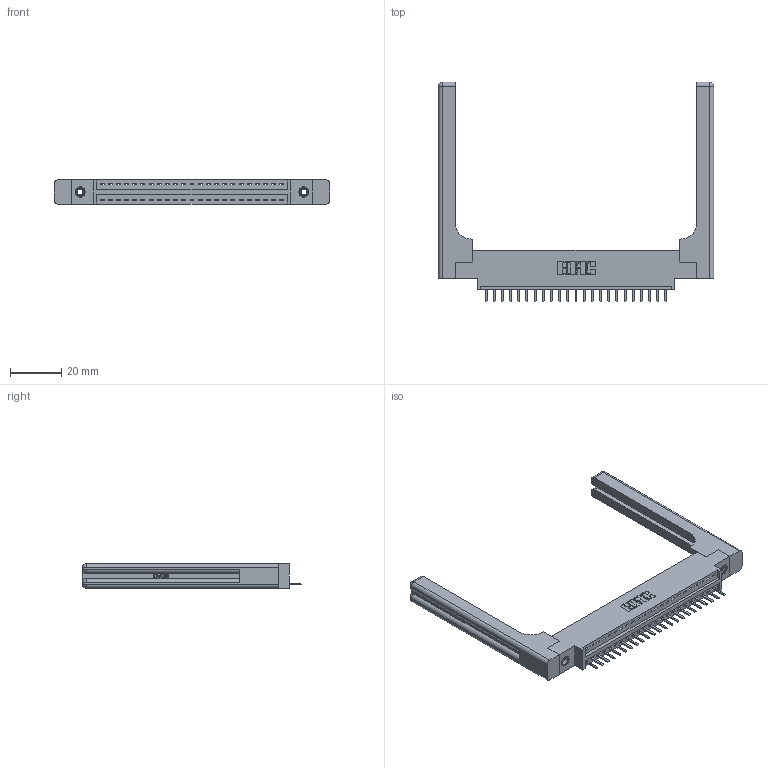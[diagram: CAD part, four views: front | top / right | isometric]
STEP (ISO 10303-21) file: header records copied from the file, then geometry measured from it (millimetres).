
FILE_DESCRIPTION (( 'STEP AP203' ), '1' );
FILE_NAME ('396-023-520-658.STEP', '2019-10-27T05:00:41', ( '' ), ( '' ), 'SwSTEP 2.0', 'SolidWorks 2016', '' );
FILE_SCHEMA (( 'CONFIG_CONTROL_DESIGN' ));
Length unit declared in the file: inch
Products named in the file (5): 396-023-520-658; 345-250-001_345-250-001-102; 345-292-001_345-293-120; 346-220-058_345-220-058; 346 Part_0.170 Offset - 0.156 Dia-TH
Assembly tree (28 placements, depth 2):
  396-023-520-658
    346 Part_0.170 Offset - 0.156 Dia-TH
    345-292-001_345-293-120  x23
    345-250-001_345-250-001-102  x2
    346-220-058_345-220-058  x2
Bounding box: 107.09 x 85.29 x 9.4 mm (x, y, z)
Volume: 17417.2 mm3; surface area: 17276.3 mm2
Topology: 28 solids, 28 shells, 1808 faces, 5239 edges, 3410 vertices
Faces by surface type: plane 1194, cylinder 554, bspline 36, cone 12, sphere 8, torus 4
Entity records: 22260 total; most frequent: CARTESIAN_POINT 4814, ORIENTED_EDGE 3556, DIRECTION 3188, EDGE_CURVE 1778, LINE 1458, VECTOR 1458, VERTEX_POINT 1174, AXIS2_PLACEMENT_3D 865
